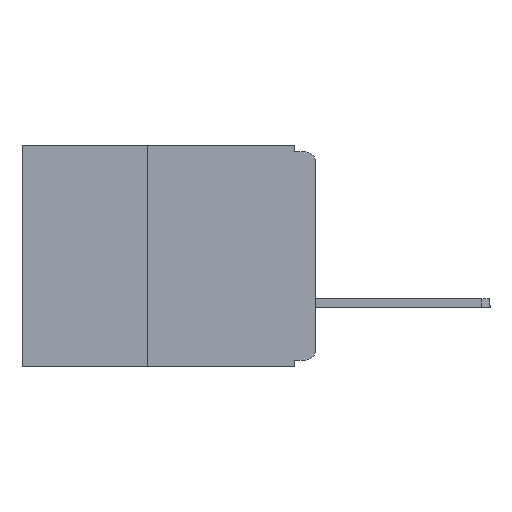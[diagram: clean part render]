
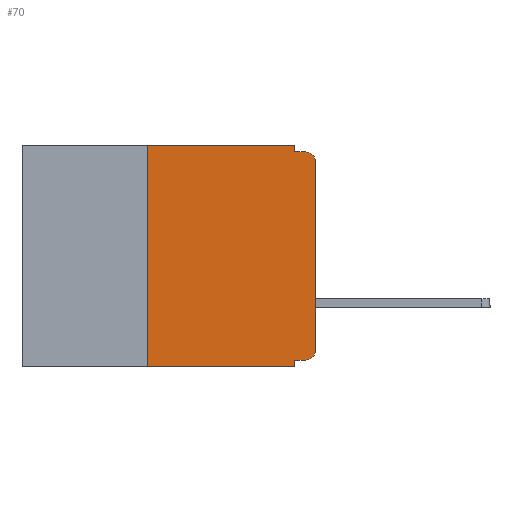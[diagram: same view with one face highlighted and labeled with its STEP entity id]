
A CAD part, left-side view. The second image highlights one B-rep face of the part: STEP entity #70.
In plain terms, the highlighted planar face has unit normal (-1, 0, 0).
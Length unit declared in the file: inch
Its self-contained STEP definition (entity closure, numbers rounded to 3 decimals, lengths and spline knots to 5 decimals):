
#50 = CARTESIAN_POINT ( 'NONE',  ( 0., 0.031, -0.32 ) ) ;
#70 = ADVANCED_FACE ( 'NONE', ( #17146 ), #22107, .F. ) ;
#472 = ORIENTED_EDGE ( 'NONE', *, *, #19852, .T. ) ;
#533 = VERTEX_POINT ( 'NONE', #50 ) ;
#605 = VERTEX_POINT ( 'NONE', #7653 ) ;
#670 = VERTEX_POINT ( 'NONE', #1774 ) ;
#824 = DIRECTION ( 'NONE',  ( 0., 0., -1. ) ) ;
#850 = CARTESIAN_POINT ( 'NONE',  ( 0., 0.25, -0.33 ) ) ;
#1243 = AXIS2_PLACEMENT_3D ( 'NONE', #12498, #2040, #14204 ) ;
#1361 = CIRCLE ( 'NONE', #1243, 0.015 ) ;
#1619 = ORIENTED_EDGE ( 'NONE', *, *, #16079, .F. ) ;
#1668 = VERTEX_POINT ( 'NONE', #8440 ) ;
#1774 = CARTESIAN_POINT ( 'NONE',  ( 0., 0.25, 0. ) ) ;
#2040 = DIRECTION ( 'NONE',  ( -1., 0., 0. ) ) ;
#2284 = CARTESIAN_POINT ( 'NONE',  ( 0., 0.031, -0.33 ) ) ;
#3121 = DIRECTION ( 'NONE',  ( 0., 0., 1. ) ) ;
#3677 = VECTOR ( 'NONE', #20665, 39.37008 ) ;
#3954 = VERTEX_POINT ( 'NONE', #21178 ) ;
#4780 = CARTESIAN_POINT ( 'NONE',  ( 0., 0.015, -0.305 ) ) ;
#5456 = VERTEX_POINT ( 'NONE', #10125 ) ;
#5525 = EDGE_LOOP ( 'NONE', ( #17851, #472, #14402, #1619, #10972, #20008, #20563, #7422, #7947, #12560 ) ) ;
#6126 = LINE ( 'NONE', #9410, #10218 ) ;
#6291 = VECTOR ( 'NONE', #15763, 39.37008 ) ;
#6544 = DIRECTION ( 'NONE',  ( 0., 0., -1. ) ) ;
#6874 = AXIS2_PLACEMENT_3D ( 'NONE', #22156, #20496, #824 ) ;
#6992 = CIRCLE ( 'NONE', #21311, 0.015 ) ;
#7139 = CARTESIAN_POINT ( 'NONE',  ( 0., 0.437, -0.33 ) ) ;
#7422 = ORIENTED_EDGE ( 'NONE', *, *, #15049, .F. ) ;
#7424 = CARTESIAN_POINT ( 'NONE',  ( 0., 0., -0.305 ) ) ;
#7653 = CARTESIAN_POINT ( 'NONE',  ( 0., 0.031, -0.33 ) ) ;
#7947 = ORIENTED_EDGE ( 'NONE', *, *, #17604, .F. ) ;
#7952 = DIRECTION ( 'NONE',  ( 0., 0., 1. ) ) ;
#8067 = CARTESIAN_POINT ( 'NONE',  ( 0., 0.437, 0. ) ) ;
#8440 = CARTESIAN_POINT ( 'NONE',  ( 0., 0.031, -0.01 ) ) ;
#8972 = VERTEX_POINT ( 'NONE', #18119 ) ;
#9410 = CARTESIAN_POINT ( 'NONE',  ( 0., 0., -0.01 ) ) ;
#9847 = DIRECTION ( 'NONE',  ( 0., -1., 0. ) ) ;
#10125 = CARTESIAN_POINT ( 'NONE',  ( 0., 0., -0.025 ) ) ;
#10218 = VECTOR ( 'NONE', #19630, 39.37008 ) ;
#10352 = VERTEX_POINT ( 'NONE', #16497 ) ;
#10928 = LINE ( 'NONE', #7139, #6291 ) ;
#10972 = ORIENTED_EDGE ( 'NONE', *, *, #22297, .F. ) ;
#10992 = LINE ( 'NONE', #19639, #11537 ) ;
#11537 = VECTOR ( 'NONE', #21365, 39.37008 ) ;
#12201 = LINE ( 'NONE', #8067, #20721 ) ;
#12388 = LINE ( 'NONE', #22358, #3677 ) ;
#12498 = CARTESIAN_POINT ( 'NONE',  ( 0., 0.015, -0.025 ) ) ;
#12560 = ORIENTED_EDGE ( 'NONE', *, *, #15322, .T. ) ;
#12618 = EDGE_CURVE ( 'NONE', #15631, #5456, #13136, .T. ) ;
#12968 = LINE ( 'NONE', #850, #16397 ) ;
#13136 = LINE ( 'NONE', #15236, #18169 ) ;
#14204 = DIRECTION ( 'NONE',  ( 0., 0., -1. ) ) ;
#14219 = EDGE_CURVE ( 'NONE', #10352, #670, #12968, .T. ) ;
#14402 = ORIENTED_EDGE ( 'NONE', *, *, #17011, .F. ) ;
#15049 = EDGE_CURVE ( 'NONE', #533, #605, #21456, .T. ) ;
#15236 = CARTESIAN_POINT ( 'NONE',  ( 0., 0., 0. ) ) ;
#15322 = EDGE_CURVE ( 'NONE', #3954, #15631, #6992, .T. ) ;
#15631 = VERTEX_POINT ( 'NONE', #7424 ) ;
#15763 = DIRECTION ( 'NONE',  ( 0., -1., 0. ) ) ;
#15995 = VERTEX_POINT ( 'NONE', #20449 ) ;
#16079 = EDGE_CURVE ( 'NONE', #8972, #1668, #12388, .T. ) ;
#16397 = VECTOR ( 'NONE', #7952, 39.37008 ) ;
#16497 = CARTESIAN_POINT ( 'NONE',  ( 0., 0.25, -0.33 ) ) ;
#16776 = DIRECTION ( 'NONE',  ( -1., 0., 0. ) ) ;
#17011 = EDGE_CURVE ( 'NONE', #1668, #15995, #6126, .T. ) ;
#17146 = FACE_OUTER_BOUND ( 'NONE', #5525, .T. ) ;
#17604 = EDGE_CURVE ( 'NONE', #3954, #533, #10992, .T. ) ;
#17837 = DIRECTION ( 'NONE',  ( 0., 0., -1. ) ) ;
#17851 = ORIENTED_EDGE ( 'NONE', *, *, #12618, .T. ) ;
#18119 = CARTESIAN_POINT ( 'NONE',  ( 0., 0.031, 0. ) ) ;
#18169 = VECTOR ( 'NONE', #3121, 39.37008 ) ;
#19630 = DIRECTION ( 'NONE',  ( 0., -1., 0. ) ) ;
#19639 = CARTESIAN_POINT ( 'NONE',  ( 0., 0., -0.32 ) ) ;
#19852 = EDGE_CURVE ( 'NONE', #5456, #15995, #1361, .T. ) ;
#20008 = ORIENTED_EDGE ( 'NONE', *, *, #14219, .F. ) ;
#20449 = CARTESIAN_POINT ( 'NONE',  ( 0., 0.015, -0.01 ) ) ;
#20496 = DIRECTION ( 'NONE',  ( 1., 0., 0. ) ) ;
#20563 = ORIENTED_EDGE ( 'NONE', *, *, #21318, .T. ) ;
#20665 = DIRECTION ( 'NONE',  ( 0., 0., -1. ) ) ;
#20721 = VECTOR ( 'NONE', #9847, 39.37008 ) ;
#20931 = VECTOR ( 'NONE', #17837, 39.37008 ) ;
#21178 = CARTESIAN_POINT ( 'NONE',  ( 0., 0.015, -0.32 ) ) ;
#21311 = AXIS2_PLACEMENT_3D ( 'NONE', #4780, #16776, #6544 ) ;
#21318 = EDGE_CURVE ( 'NONE', #10352, #605, #10928, .T. ) ;
#21365 = DIRECTION ( 'NONE',  ( 0., 1., 0. ) ) ;
#21456 = LINE ( 'NONE', #2284, #20931 ) ;
#22107 = PLANE ( 'NONE',  #6874 ) ;
#22156 = CARTESIAN_POINT ( 'NONE',  ( 0., 0.437, 0. ) ) ;
#22297 = EDGE_CURVE ( 'NONE', #670, #8972, #12201, .T. ) ;
#22358 = CARTESIAN_POINT ( 'NONE',  ( 0., 0.031, 0. ) ) ;
